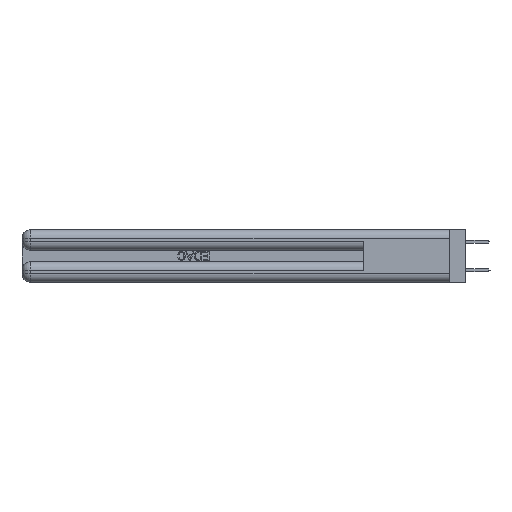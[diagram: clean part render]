
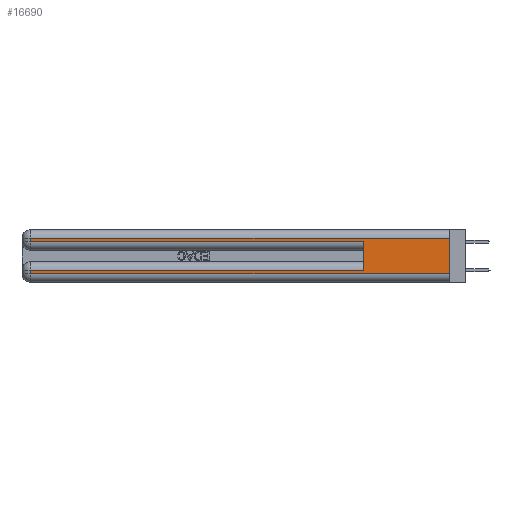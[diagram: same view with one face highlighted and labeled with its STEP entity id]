
A CAD part, left-side view. The second image highlights one B-rep face of the part: STEP entity #16690.
In plain terms, the highlighted planar face has unit normal (-1, 0, 0).
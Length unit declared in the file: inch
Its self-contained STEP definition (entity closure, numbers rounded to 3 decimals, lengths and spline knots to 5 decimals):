
#705 = CARTESIAN_POINT ( 'NONE',  ( 0., 2.94, 0.085 ) ) ;
#1036 = LINE ( 'NONE', #36962, #8263 ) ;
#1517 = ORIENTED_EDGE ( 'NONE', *, *, #36348, .T. ) ;
#2001 = VERTEX_POINT ( 'NONE', #705 ) ;
#2087 = DIRECTION ( 'NONE',  ( 0., 0., -1. ) ) ;
#2175 = LINE ( 'NONE', #6680, #5076 ) ;
#2603 = CARTESIAN_POINT ( 'NONE',  ( 0., 0., 0.285 ) ) ;
#3453 = EDGE_CURVE ( 'NONE', #2001, #38055, #8764, .T. ) ;
#4689 = VERTEX_POINT ( 'NONE', #20401 ) ;
#5076 = VECTOR ( 'NONE', #25063, 39.37008 ) ;
#6326 = LINE ( 'NONE', #20459, #22606 ) ;
#6554 = CARTESIAN_POINT ( 'NONE',  ( 0., 0., 0.31 ) ) ;
#6680 = CARTESIAN_POINT ( 'NONE',  ( 0., 0.6, 0.145 ) ) ;
#6759 = VECTOR ( 'NONE', #30240, 39.37008 ) ;
#6997 = DIRECTION ( 'NONE',  ( 1., 0., 0. ) ) ;
#8263 = VECTOR ( 'NONE', #21708, 39.37008 ) ;
#8764 = LINE ( 'NONE', #10976, #16889 ) ;
#9665 = EDGE_CURVE ( 'NONE', #38055, #12218, #1036, .T. ) ;
#9920 = PLANE ( 'NONE',  #14626 ) ;
#10148 = DIRECTION ( 'NONE',  ( 0., 1., 0. ) ) ;
#10976 = CARTESIAN_POINT ( 'NONE',  ( 0., 2.94, 0.37 ) ) ;
#12218 = VERTEX_POINT ( 'NONE', #32185 ) ;
#12246 = EDGE_LOOP ( 'NONE', ( #22390, #35431, #16567, #1517, #22381, #18266, #14139, #30115 ) ) ;
#12793 = VECTOR ( 'NONE', #38797, 39.37008 ) ;
#13347 = VERTEX_POINT ( 'NONE', #22830 ) ;
#14139 = ORIENTED_EDGE ( 'NONE', *, *, #3453, .T. ) ;
#14384 = EDGE_CURVE ( 'NONE', #4689, #13347, #28549, .T. ) ;
#14626 = AXIS2_PLACEMENT_3D ( 'NONE', #16083, #6997, #28444 ) ;
#16083 = CARTESIAN_POINT ( 'NONE',  ( 0., 0., 0.37 ) ) ;
#16327 = CARTESIAN_POINT ( 'NONE',  ( 0., 0.6, 0.285 ) ) ;
#16567 = ORIENTED_EDGE ( 'NONE', *, *, #32958, .T. ) ;
#16690 = ADVANCED_FACE ( 'NONE', ( #36488 ), #9920, .F. ) ;
#16889 = VECTOR ( 'NONE', #26317, 39.37008 ) ;
#18266 = ORIENTED_EDGE ( 'NONE', *, *, #38666, .T. ) ;
#20401 = CARTESIAN_POINT ( 'NONE',  ( 0., 0., 0.31 ) ) ;
#20459 = CARTESIAN_POINT ( 'NONE',  ( 0., 0., 0.37 ) ) ;
#21708 = DIRECTION ( 'NONE',  ( 0., -1., 0. ) ) ;
#22381 = ORIENTED_EDGE ( 'NONE', *, *, #33283, .F. ) ;
#22390 = ORIENTED_EDGE ( 'NONE', *, *, #35622, .F. ) ;
#22444 = CARTESIAN_POINT ( 'NONE',  ( 0., 2.94, 0.06 ) ) ;
#22606 = VECTOR ( 'NONE', #2087, 39.37008 ) ;
#22767 = VERTEX_POINT ( 'NONE', #31136 ) ;
#22830 = CARTESIAN_POINT ( 'NONE',  ( 0., 2.94, 0.31 ) ) ;
#24177 = VECTOR ( 'NONE', #10148, 39.37008 ) ;
#24585 = VERTEX_POINT ( 'NONE', #33627 ) ;
#25063 = DIRECTION ( 'NONE',  ( 0., 0., 1. ) ) ;
#26004 = VERTEX_POINT ( 'NONE', #16327 ) ;
#26317 = DIRECTION ( 'NONE',  ( 0., 0., -1. ) ) ;
#28444 = DIRECTION ( 'NONE',  ( 0., 0., -1. ) ) ;
#28547 = CARTESIAN_POINT ( 'NONE',  ( 0., 0., 0.085 ) ) ;
#28549 = LINE ( 'NONE', #6554, #30498 ) ;
#30115 = ORIENTED_EDGE ( 'NONE', *, *, #9665, .T. ) ;
#30240 = DIRECTION ( 'NONE',  ( 0., -1., 0. ) ) ;
#30498 = VECTOR ( 'NONE', #37080, 39.37008 ) ;
#31136 = CARTESIAN_POINT ( 'NONE',  ( 0., 2.94, 0.285 ) ) ;
#31358 = LINE ( 'NONE', #28547, #24177 ) ;
#32185 = CARTESIAN_POINT ( 'NONE',  ( 0., 0., 0.06 ) ) ;
#32958 = EDGE_CURVE ( 'NONE', #13347, #22767, #37220, .T. ) ;
#33283 = EDGE_CURVE ( 'NONE', #24585, #26004, #2175, .T. ) ;
#33627 = CARTESIAN_POINT ( 'NONE',  ( 0., 0.6, 0.085 ) ) ;
#35431 = ORIENTED_EDGE ( 'NONE', *, *, #14384, .T. ) ;
#35622 = EDGE_CURVE ( 'NONE', #4689, #12218, #6326, .T. ) ;
#35900 = CARTESIAN_POINT ( 'NONE',  ( 0., 2.94, 0.37 ) ) ;
#36348 = EDGE_CURVE ( 'NONE', #22767, #26004, #39305, .T. ) ;
#36488 = FACE_OUTER_BOUND ( 'NONE', #12246, .T. ) ;
#36962 = CARTESIAN_POINT ( 'NONE',  ( 0., 0., 0.06 ) ) ;
#37080 = DIRECTION ( 'NONE',  ( 0., 1., 0. ) ) ;
#37220 = LINE ( 'NONE', #35900, #12793 ) ;
#38055 = VERTEX_POINT ( 'NONE', #22444 ) ;
#38666 = EDGE_CURVE ( 'NONE', #24585, #2001, #31358, .T. ) ;
#38797 = DIRECTION ( 'NONE',  ( 0., 0., -1. ) ) ;
#39305 = LINE ( 'NONE', #2603, #6759 ) ;
